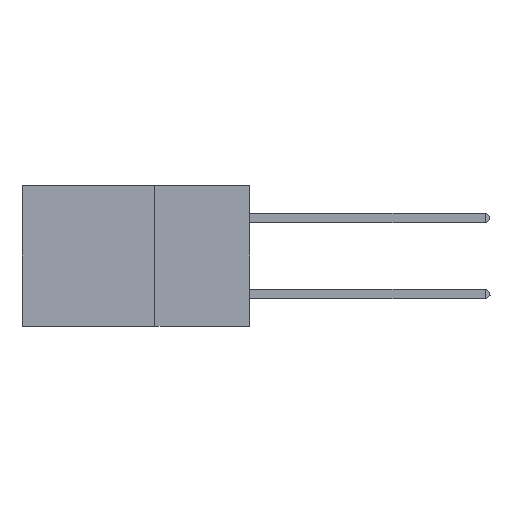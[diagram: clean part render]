
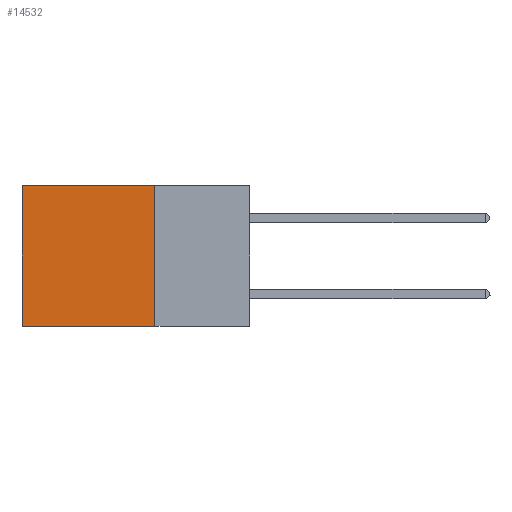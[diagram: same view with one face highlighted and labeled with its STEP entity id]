
A CAD part, left-side view. The second image highlights one B-rep face of the part: STEP entity #14532.
In plain terms, the highlighted planar face has unit normal (-1, 0, 0).
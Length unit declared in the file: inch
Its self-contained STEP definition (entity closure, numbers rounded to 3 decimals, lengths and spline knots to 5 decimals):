
#132 = LINE ( 'NONE', #36812, #36915 ) ;
#1923 = CARTESIAN_POINT ( 'NONE',  ( 0.2875, 0.25, -0.37 ) ) ;
#3598 = CARTESIAN_POINT ( 'NONE',  ( 0.2875, 0.25, 0. ) ) ;
#5233 = ORIENTED_EDGE ( 'NONE', *, *, #11207, .T. ) ;
#5702 = CARTESIAN_POINT ( 'NONE',  ( 0.2875, 0.6, -0.37 ) ) ;
#6077 = VERTEX_POINT ( 'NONE', #6440 ) ;
#6440 = CARTESIAN_POINT ( 'NONE',  ( 0.2875, 0.25, -0.37 ) ) ;
#7647 = ORIENTED_EDGE ( 'NONE', *, *, #10166, .F. ) ;
#8386 = EDGE_CURVE ( 'NONE', #13201, #6077, #132, .T. ) ;
#9852 = DIRECTION ( 'NONE',  ( 1., 0., 0. ) ) ;
#10166 = EDGE_CURVE ( 'NONE', #6077, #12375, #10820, .T. ) ;
#10820 = LINE ( 'NONE', #1923, #15429 ) ;
#11207 = EDGE_CURVE ( 'NONE', #24104, #12375, #33943, .T. ) ;
#11943 = CARTESIAN_POINT ( 'NONE',  ( 0.2875, 0.25, 0. ) ) ;
#12190 = DIRECTION ( 'NONE',  ( 0., 1., 0. ) ) ;
#12375 = VERTEX_POINT ( 'NONE', #5702 ) ;
#12666 = VECTOR ( 'NONE', #19942, 39.37008 ) ;
#13201 = VERTEX_POINT ( 'NONE', #28226 ) ;
#14532 = ADVANCED_FACE ( 'NONE', ( #16533 ), #35501, .F. ) ;
#14727 = AXIS2_PLACEMENT_3D ( 'NONE', #3598, #9852, #33038 ) ;
#15429 = VECTOR ( 'NONE', #19536, 39.37008 ) ;
#16533 = FACE_OUTER_BOUND ( 'NONE', #23228, .T. ) ;
#17042 = CARTESIAN_POINT ( 'NONE',  ( 0.2875, 0.6, 0. ) ) ;
#19536 = DIRECTION ( 'NONE',  ( 0., 1., 0. ) ) ;
#19942 = DIRECTION ( 'NONE',  ( 0., 0., -1. ) ) ;
#20758 = CARTESIAN_POINT ( 'NONE',  ( 0.2875, 0.6, 0. ) ) ;
#22670 = ORIENTED_EDGE ( 'NONE', *, *, #31402, .T. ) ;
#23228 = EDGE_LOOP ( 'NONE', ( #5233, #7647, #27782, #22670 ) ) ;
#24104 = VERTEX_POINT ( 'NONE', #20758 ) ;
#27643 = VECTOR ( 'NONE', #12190, 39.37008 ) ;
#27782 = ORIENTED_EDGE ( 'NONE', *, *, #8386, .F. ) ;
#28226 = CARTESIAN_POINT ( 'NONE',  ( 0.2875, 0.25, 0. ) ) ;
#29860 = LINE ( 'NONE', #11943, #27643 ) ;
#31402 = EDGE_CURVE ( 'NONE', #13201, #24104, #29860, .T. ) ;
#33038 = DIRECTION ( 'NONE',  ( 0., 0., -1. ) ) ;
#33943 = LINE ( 'NONE', #17042, #12666 ) ;
#35501 = PLANE ( 'NONE',  #14727 ) ;
#35980 = DIRECTION ( 'NONE',  ( 0., 0., -1. ) ) ;
#36812 = CARTESIAN_POINT ( 'NONE',  ( 0.2875, 0.25, 0. ) ) ;
#36915 = VECTOR ( 'NONE', #35980, 39.37008 ) ;
